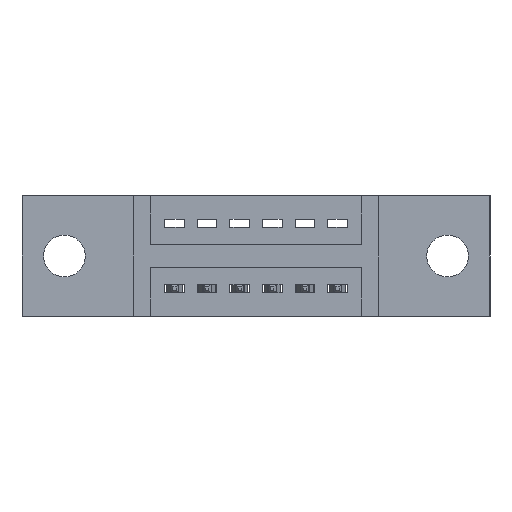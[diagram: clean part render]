
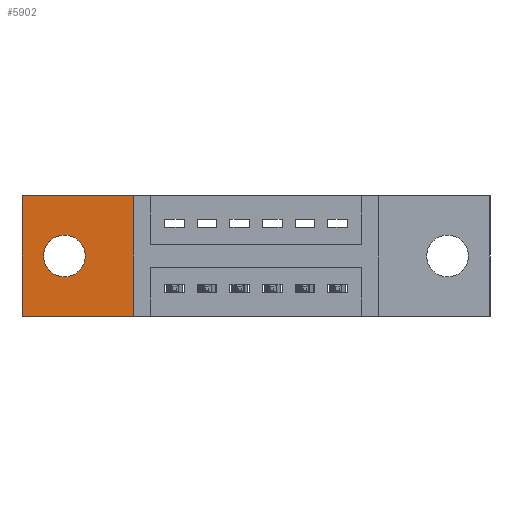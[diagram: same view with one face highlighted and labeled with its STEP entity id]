
A CAD part, front view. The second image highlights one B-rep face of the part: STEP entity #5902.
In plain terms, the highlighted planar face has unit normal (0, -1, 0).
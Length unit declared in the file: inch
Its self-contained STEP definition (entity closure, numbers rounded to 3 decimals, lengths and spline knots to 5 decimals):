
#293 = LINE ( 'NONE', #7657, #386 ) ;
#386 = VECTOR ( 'NONE', #4717, 39.37008 ) ;
#414 = CARTESIAN_POINT ( 'NONE',  ( 0.13, 0.17, -0.185 ) ) ;
#510 = EDGE_LOOP ( 'NONE', ( #2028, #4804, #6581, #6871 ) ) ;
#1077 = DIRECTION ( 'NONE',  ( 0., 0., -1. ) ) ;
#1169 = EDGE_LOOP ( 'NONE', ( #7218, #5959 ) ) ;
#1377 = CARTESIAN_POINT ( 'NONE',  ( 0., 0.17, -0.37 ) ) ;
#1501 = VECTOR ( 'NONE', #8303, 39.37008 ) ;
#1694 = CARTESIAN_POINT ( 'NONE',  ( 0.3425, 0.17, 0. ) ) ;
#1866 = DIRECTION ( 'NONE',  ( 0., 0., -1. ) ) ;
#2028 = ORIENTED_EDGE ( 'NONE', *, *, #8799, .T. ) ;
#2070 = CIRCLE ( 'NONE', #5432, 0.064 ) ;
#2118 = FACE_BOUND ( 'NONE', #1169, .T. ) ;
#2299 = EDGE_CURVE ( 'NONE', #4452, #4414, #2070, .T. ) ;
#2613 = FACE_OUTER_BOUND ( 'NONE', #510, .T. ) ;
#2815 = VERTEX_POINT ( 'NONE', #3551 ) ;
#2821 = VECTOR ( 'NONE', #4864, 39.37008 ) ;
#3551 = CARTESIAN_POINT ( 'NONE',  ( 0.3425, 0.17, -0.37 ) ) ;
#4130 = CARTESIAN_POINT ( 'NONE',  ( 0.3425, 0.17, 0. ) ) ;
#4176 = LINE ( 'NONE', #8161, #2821 ) ;
#4414 = VERTEX_POINT ( 'NONE', #6682 ) ;
#4452 = VERTEX_POINT ( 'NONE', #9162 ) ;
#4717 = DIRECTION ( 'NONE',  ( -1., 0., 0. ) ) ;
#4804 = ORIENTED_EDGE ( 'NONE', *, *, #8286, .T. ) ;
#4864 = DIRECTION ( 'NONE',  ( 1., 0., 0. ) ) ;
#4943 = CARTESIAN_POINT ( 'NONE',  ( 0., 0.17, 0. ) ) ;
#5112 = CARTESIAN_POINT ( 'NONE',  ( 0., 0.17, -0.37 ) ) ;
#5295 = CIRCLE ( 'NONE', #6926, 0.064 ) ;
#5432 = AXIS2_PLACEMENT_3D ( 'NONE', #9228, #5536, #1077 ) ;
#5536 = DIRECTION ( 'NONE',  ( 0., -1., 0. ) ) ;
#5562 = DIRECTION ( 'NONE',  ( 0., -1., 0. ) ) ;
#5762 = DIRECTION ( 'NONE',  ( 0., 0., -1. ) ) ;
#5825 = PLANE ( 'NONE',  #5940 ) ;
#5902 = ADVANCED_FACE ( 'NONE', ( #2118, #2613 ), #5825, .T. ) ;
#5940 = AXIS2_PLACEMENT_3D ( 'NONE', #1377, #6421, #5762 ) ;
#5959 = ORIENTED_EDGE ( 'NONE', *, *, #9043, .F. ) ;
#6236 = EDGE_CURVE ( 'NONE', #2815, #9049, #8239, .T. ) ;
#6280 = EDGE_CURVE ( 'NONE', #9049, #9489, #293, .T. ) ;
#6421 = DIRECTION ( 'NONE',  ( 0., -1., 0. ) ) ;
#6581 = ORIENTED_EDGE ( 'NONE', *, *, #6236, .T. ) ;
#6653 = VECTOR ( 'NONE', #9381, 39.37008 ) ;
#6682 = CARTESIAN_POINT ( 'NONE',  ( 0.13, 0.17, -0.249 ) ) ;
#6871 = ORIENTED_EDGE ( 'NONE', *, *, #6280, .T. ) ;
#6926 = AXIS2_PLACEMENT_3D ( 'NONE', #414, #5562, #1866 ) ;
#7218 = ORIENTED_EDGE ( 'NONE', *, *, #2299, .F. ) ;
#7657 = CARTESIAN_POINT ( 'NONE',  ( 0., 0.17, 0. ) ) ;
#7830 = LINE ( 'NONE', #4943, #6653 ) ;
#8161 = CARTESIAN_POINT ( 'NONE',  ( 0., 0.17, -0.37 ) ) ;
#8239 = LINE ( 'NONE', #1694, #1501 ) ;
#8286 = EDGE_CURVE ( 'NONE', #9165, #2815, #4176, .T. ) ;
#8303 = DIRECTION ( 'NONE',  ( 0., 0., 1. ) ) ;
#8451 = CARTESIAN_POINT ( 'NONE',  ( 0., 0.17, 0. ) ) ;
#8799 = EDGE_CURVE ( 'NONE', #9489, #9165, #7830, .T. ) ;
#9043 = EDGE_CURVE ( 'NONE', #4414, #4452, #5295, .T. ) ;
#9049 = VERTEX_POINT ( 'NONE', #4130 ) ;
#9162 = CARTESIAN_POINT ( 'NONE',  ( 0.13, 0.17, -0.121 ) ) ;
#9165 = VERTEX_POINT ( 'NONE', #5112 ) ;
#9228 = CARTESIAN_POINT ( 'NONE',  ( 0.13, 0.17, -0.185 ) ) ;
#9381 = DIRECTION ( 'NONE',  ( 0., 0., -1. ) ) ;
#9489 = VERTEX_POINT ( 'NONE', #8451 ) ;
